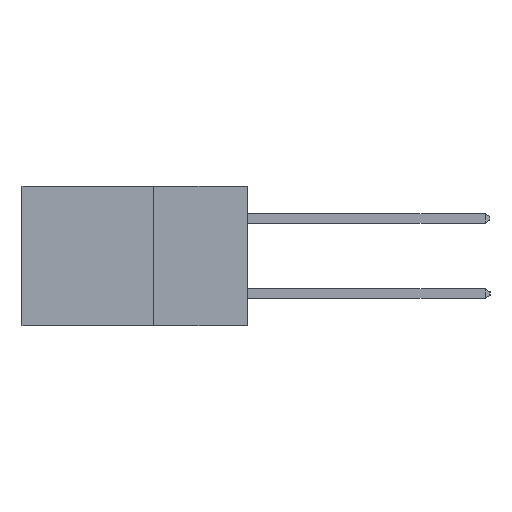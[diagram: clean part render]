
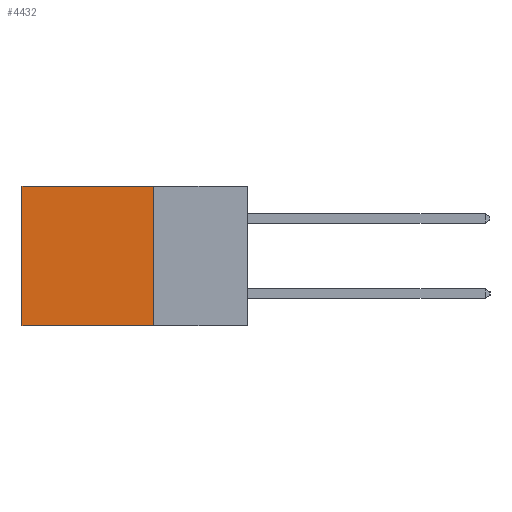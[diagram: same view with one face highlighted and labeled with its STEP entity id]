
A CAD part, left-side view. The second image highlights one B-rep face of the part: STEP entity #4432.
In plain terms, the highlighted planar face has unit normal (-1, 0, 0).
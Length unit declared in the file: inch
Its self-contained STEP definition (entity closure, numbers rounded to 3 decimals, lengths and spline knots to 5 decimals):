
#268 = CARTESIAN_POINT ( 'NONE',  ( 0.2615, 0.25, 0. ) ) ;
#945 = EDGE_CURVE ( 'NONE', #11821, #9481, #11043, .T. ) ;
#983 = CARTESIAN_POINT ( 'NONE',  ( 0.2615, 0.25, -0.37 ) ) ;
#1266 = ORIENTED_EDGE ( 'NONE', *, *, #2932, .F. ) ;
#1382 = VECTOR ( 'NONE', #1418, 39.37008 ) ;
#1418 = DIRECTION ( 'NONE',  ( 0., 0., -1. ) ) ;
#1468 = CARTESIAN_POINT ( 'NONE',  ( 0.2615, 0.6, -0.37 ) ) ;
#1673 = LINE ( 'NONE', #5753, #7145 ) ;
#2333 = FACE_OUTER_BOUND ( 'NONE', #10687, .T. ) ;
#2932 = EDGE_CURVE ( 'NONE', #9481, #10994, #1673, .T. ) ;
#4432 = ADVANCED_FACE ( 'NONE', ( #2333 ), #7276, .F. ) ;
#4942 = DIRECTION ( 'NONE',  ( 0., 1., 0. ) ) ;
#5180 = CARTESIAN_POINT ( 'NONE',  ( 0.2615, 0.6, 0. ) ) ;
#5541 = LINE ( 'NONE', #10620, #10655 ) ;
#5753 = CARTESIAN_POINT ( 'NONE',  ( 0.2615, 0.25, -0.37 ) ) ;
#6810 = ORIENTED_EDGE ( 'NONE', *, *, #10639, .T. ) ;
#7145 = VECTOR ( 'NONE', #4942, 39.37008 ) ;
#7185 = LINE ( 'NONE', #1468, #1382 ) ;
#7193 = DIRECTION ( 'NONE',  ( 0., 0., -1. ) ) ;
#7249 = DIRECTION ( 'NONE',  ( 1., 0., 0. ) ) ;
#7276 = PLANE ( 'NONE',  #10711 ) ;
#7325 = CARTESIAN_POINT ( 'NONE',  ( 0.2615, 0.25, -0.37 ) ) ;
#8019 = VECTOR ( 'NONE', #11253, 39.37008 ) ;
#8030 = CARTESIAN_POINT ( 'NONE',  ( 0.2615, 0.6, -0.37 ) ) ;
#8680 = EDGE_CURVE ( 'NONE', #10436, #10994, #7185, .T. ) ;
#9481 = VERTEX_POINT ( 'NONE', #9700 ) ;
#9700 = CARTESIAN_POINT ( 'NONE',  ( 0.2615, 0.25, -0.37 ) ) ;
#10436 = VERTEX_POINT ( 'NONE', #5180 ) ;
#10620 = CARTESIAN_POINT ( 'NONE',  ( 0.2615, 0.25, 0. ) ) ;
#10639 = EDGE_CURVE ( 'NONE', #11821, #10436, #5541, .T. ) ;
#10655 = VECTOR ( 'NONE', #11668, 39.37008 ) ;
#10687 = EDGE_LOOP ( 'NONE', ( #12879, #1266, #13209, #6810 ) ) ;
#10711 = AXIS2_PLACEMENT_3D ( 'NONE', #7325, #7249, #7193 ) ;
#10994 = VERTEX_POINT ( 'NONE', #8030 ) ;
#11043 = LINE ( 'NONE', #983, #8019 ) ;
#11253 = DIRECTION ( 'NONE',  ( 0., 0., -1. ) ) ;
#11668 = DIRECTION ( 'NONE',  ( 0., 1., 0. ) ) ;
#11821 = VERTEX_POINT ( 'NONE', #268 ) ;
#12879 = ORIENTED_EDGE ( 'NONE', *, *, #8680, .T. ) ;
#13209 = ORIENTED_EDGE ( 'NONE', *, *, #945, .F. ) ;
